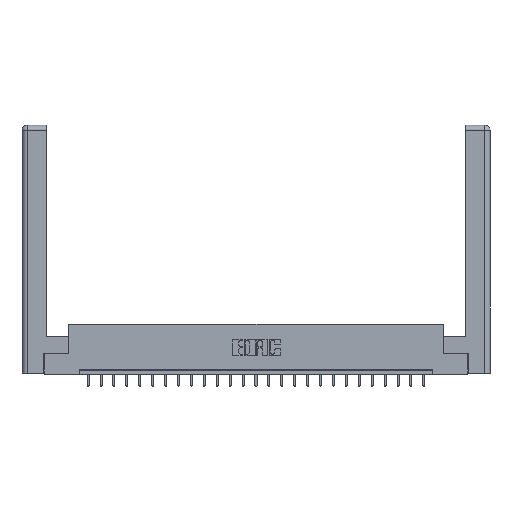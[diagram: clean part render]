
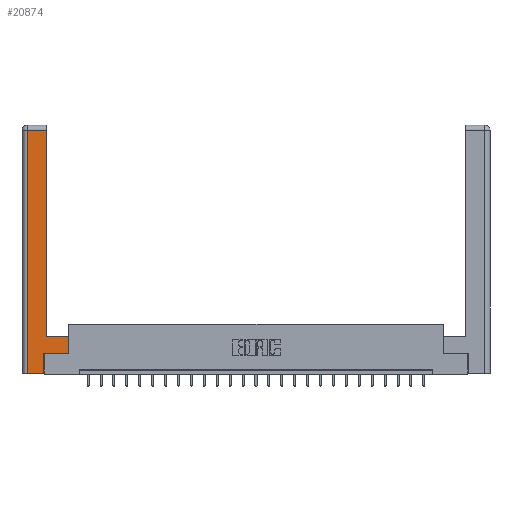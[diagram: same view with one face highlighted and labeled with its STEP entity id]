
A CAD part, top view. The second image highlights one B-rep face of the part: STEP entity #20874.
In plain terms, the highlighted planar face has unit normal (0, 0, 1).
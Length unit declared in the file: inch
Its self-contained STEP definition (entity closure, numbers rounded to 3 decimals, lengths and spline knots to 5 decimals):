
#1449 = CARTESIAN_POINT ( 'NONE',  ( 0.565, 0.245, 0. ) ) ;
#2037 = CARTESIAN_POINT ( 'NONE',  ( 0., 0., 0. ) ) ;
#2131 = ORIENTED_EDGE ( 'NONE', *, *, #8165, .T. ) ;
#2621 = DIRECTION ( 'NONE',  ( 0., 1., 0. ) ) ;
#2981 = FACE_OUTER_BOUND ( 'NONE', #20295, .T. ) ;
#3612 = DIRECTION ( 'NONE',  ( -1., 0., 0. ) ) ;
#3987 = EDGE_CURVE ( 'NONE', #4252, #18190, #4132, .T. ) ;
#4132 = LINE ( 'NONE', #17866, #23852 ) ;
#4215 = VERTEX_POINT ( 'NONE', #1449 ) ;
#4252 = VERTEX_POINT ( 'NONE', #5198 ) ;
#4378 = CARTESIAN_POINT ( 'NONE',  ( 0.265, 0.245, 0. ) ) ;
#4685 = CARTESIAN_POINT ( 'NONE',  ( 0.295, 0.45, 0. ) ) ;
#4877 = VERTEX_POINT ( 'NONE', #10077 ) ;
#4893 = CARTESIAN_POINT ( 'NONE',  ( 0.295, 2.94, 0. ) ) ;
#4915 = CARTESIAN_POINT ( 'NONE',  ( 0.0615, 2.94, 0. ) ) ;
#5059 = CARTESIAN_POINT ( 'NONE',  ( 0.565, 0.45, 0. ) ) ;
#5198 = CARTESIAN_POINT ( 'NONE',  ( 0.265, 0., 0. ) ) ;
#6306 = ORIENTED_EDGE ( 'NONE', *, *, #3987, .T. ) ;
#6350 = LINE ( 'NONE', #17448, #9011 ) ;
#6451 = DIRECTION ( 'NONE',  ( 0., 1., 0. ) ) ;
#6831 = DIRECTION ( 'NONE',  ( -1., 0., 0. ) ) ;
#7447 = PLANE ( 'NONE',  #19668 ) ;
#7450 = VECTOR ( 'NONE', #21946, 39.37008 ) ;
#8155 = DIRECTION ( 'NONE',  ( 1., 0., 0. ) ) ;
#8165 = EDGE_CURVE ( 'NONE', #4877, #19592, #17586, .T. ) ;
#8173 = VERTEX_POINT ( 'NONE', #4893 ) ;
#8643 = LINE ( 'NONE', #10206, #11916 ) ;
#9011 = VECTOR ( 'NONE', #22834, 39.37008 ) ;
#9091 = ORIENTED_EDGE ( 'NONE', *, *, #12384, .T. ) ;
#9116 = CARTESIAN_POINT ( 'NONE',  ( 0.295, 0.45, 0. ) ) ;
#9211 = VECTOR ( 'NONE', #2621, 39.37008 ) ;
#9926 = ORIENTED_EDGE ( 'NONE', *, *, #23911, .T. ) ;
#10015 = EDGE_CURVE ( 'NONE', #4215, #24664, #6350, .T. ) ;
#10077 = CARTESIAN_POINT ( 'NONE',  ( 0.0615, 2.94, 0. ) ) ;
#10206 = CARTESIAN_POINT ( 'NONE',  ( 0.265, 0., 0. ) ) ;
#11230 = EDGE_CURVE ( 'NONE', #19592, #4252, #8643, .T. ) ;
#11916 = VECTOR ( 'NONE', #23367, 39.37008 ) ;
#12046 = CARTESIAN_POINT ( 'NONE',  ( 0.565, 0.245, 0. ) ) ;
#12140 = DIRECTION ( 'NONE',  ( -1., 0., 0. ) ) ;
#12384 = EDGE_CURVE ( 'NONE', #8173, #4877, #21968, .T. ) ;
#13999 = CARTESIAN_POINT ( 'NONE',  ( 0.295, 3., 0. ) ) ;
#14267 = LINE ( 'NONE', #13999, #9211 ) ;
#14883 = EDGE_CURVE ( 'NONE', #18190, #4215, #15982, .T. ) ;
#15818 = ORIENTED_EDGE ( 'NONE', *, *, #10015, .T. ) ;
#15982 = LINE ( 'NONE', #12046, #20183 ) ;
#17448 = CARTESIAN_POINT ( 'NONE',  ( 0.565, 0.45, 0. ) ) ;
#17484 = EDGE_CURVE ( 'NONE', #24664, #19121, #18899, .T. ) ;
#17586 = LINE ( 'NONE', #22106, #7450 ) ;
#17704 = ORIENTED_EDGE ( 'NONE', *, *, #14883, .T. ) ;
#17866 = CARTESIAN_POINT ( 'NONE',  ( 0.265, 0.245, 0. ) ) ;
#18112 = ORIENTED_EDGE ( 'NONE', *, *, #17484, .T. ) ;
#18190 = VERTEX_POINT ( 'NONE', #4378 ) ;
#18899 = LINE ( 'NONE', #4685, #23053 ) ;
#19121 = VERTEX_POINT ( 'NONE', #9116 ) ;
#19141 = DIRECTION ( 'NONE',  ( 0., 0., -1. ) ) ;
#19592 = VERTEX_POINT ( 'NONE', #20445 ) ;
#19668 = AXIS2_PLACEMENT_3D ( 'NONE', #2037, #19141, #3612 ) ;
#20099 = ORIENTED_EDGE ( 'NONE', *, *, #11230, .T. ) ;
#20183 = VECTOR ( 'NONE', #8155, 39.37008 ) ;
#20295 = EDGE_LOOP ( 'NONE', ( #9926, #9091, #2131, #20099, #6306, #17704, #15818, #18112 ) ) ;
#20445 = CARTESIAN_POINT ( 'NONE',  ( 0.0615, 0., 0. ) ) ;
#20874 = ADVANCED_FACE ( 'NONE', ( #2981 ), #7447, .F. ) ;
#21946 = DIRECTION ( 'NONE',  ( 0., -1., 0. ) ) ;
#21968 = LINE ( 'NONE', #4915, #24060 ) ;
#22106 = CARTESIAN_POINT ( 'NONE',  ( 0.0615, 0., 0. ) ) ;
#22834 = DIRECTION ( 'NONE',  ( 0., 1., 0. ) ) ;
#23053 = VECTOR ( 'NONE', #12140, 39.37008 ) ;
#23367 = DIRECTION ( 'NONE',  ( 1., 0., 0. ) ) ;
#23852 = VECTOR ( 'NONE', #6451, 39.37008 ) ;
#23911 = EDGE_CURVE ( 'NONE', #19121, #8173, #14267, .T. ) ;
#24060 = VECTOR ( 'NONE', #6831, 39.37008 ) ;
#24664 = VERTEX_POINT ( 'NONE', #5059 ) ;
